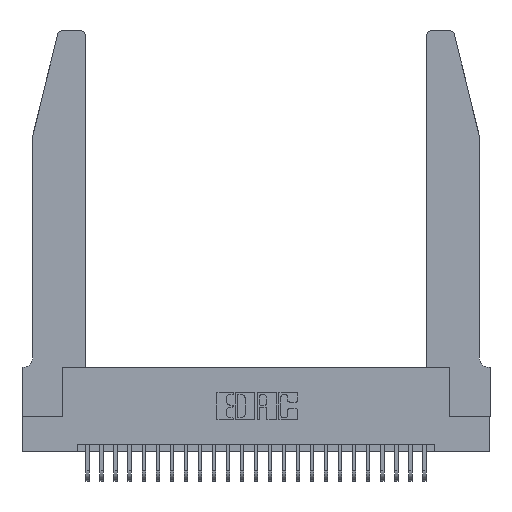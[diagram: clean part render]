
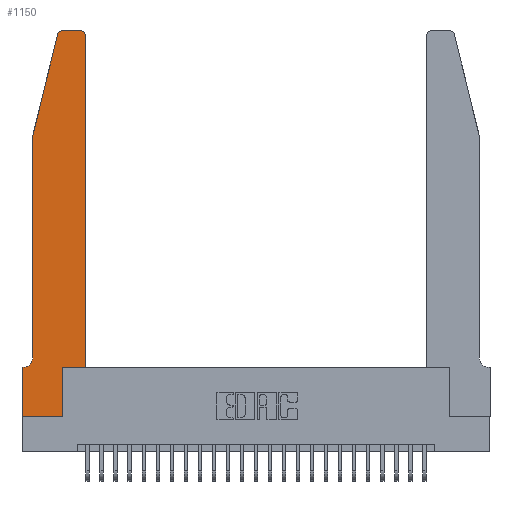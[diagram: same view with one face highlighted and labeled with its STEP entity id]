
A CAD part, top view. The second image highlights one B-rep face of the part: STEP entity #1150.
In plain terms, the highlighted planar face has unit normal (0, 0, 1).
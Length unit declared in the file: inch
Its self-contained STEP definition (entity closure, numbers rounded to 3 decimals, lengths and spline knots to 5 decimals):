
#134 = CARTESIAN_POINT ( 'NONE',  ( 0.2865, 0.35, 0.37 ) ) ;
#166 = ORIENTED_EDGE ( 'NONE', *, *, #511, .T. ) ;
#240 = CARTESIAN_POINT ( 'NONE',  ( 0.4205, 2.72, 0.37 ) ) ;
#432 = DIRECTION ( 'NONE',  ( 0., 0., 1. ) ) ;
#511 = EDGE_CURVE ( 'NONE', #27506, #2428, #8709, .T. ) ;
#896 = CARTESIAN_POINT ( 'NONE',  ( 0., 0., 0.37 ) ) ;
#1150 = ADVANCED_FACE ( 'NONE', ( #13424 ), #23059, .T. ) ;
#1518 = DIRECTION ( 'NONE',  ( 0., -1., 0. ) ) ;
#2144 = VERTEX_POINT ( 'NONE', #25174 ) ;
#2336 = VERTEX_POINT ( 'NONE', #21689 ) ;
#2428 = VERTEX_POINT ( 'NONE', #3837 ) ;
#2431 = CARTESIAN_POINT ( 'NONE',  ( 0., 0., 0.37 ) ) ;
#2516 = EDGE_CURVE ( 'NONE', #2428, #14756, #23964, .T. ) ;
#2703 = CARTESIAN_POINT ( 'NONE',  ( 0.2865, 0., 0.37 ) ) ;
#2908 = DIRECTION ( 'NONE',  ( 1., 0., 0. ) ) ;
#3651 = DIRECTION ( 'NONE',  ( -0.239, -0.971, 0. ) ) ;
#3837 = CARTESIAN_POINT ( 'NONE',  ( 0.4505, 0.35, 0.37 ) ) ;
#4097 = ORIENTED_EDGE ( 'NONE', *, *, #15264, .T. ) ;
#4547 = EDGE_CURVE ( 'NONE', #18676, #14718, #15716, .T. ) ;
#4570 = DIRECTION ( 'NONE',  ( 0., 1., 0. ) ) ;
#4845 = DIRECTION ( 'NONE',  ( 1., 0., 0. ) ) ;
#5157 = VERTEX_POINT ( 'NONE', #12170 ) ;
#5263 = DIRECTION ( 'NONE',  ( 1., 0., 0. ) ) ;
#5652 = DIRECTION ( 'NONE',  ( 1., 0., 0. ) ) ;
#6061 = LINE ( 'NONE', #9587, #26533 ) ;
#6070 = EDGE_CURVE ( 'NONE', #5157, #25349, #18004, .T. ) ;
#6197 = DIRECTION ( 'NONE',  ( 0., 0., 1. ) ) ;
#6421 = CARTESIAN_POINT ( 'NONE',  ( 0.4505, 0.35, 0.37 ) ) ;
#6541 = DIRECTION ( 'NONE',  ( 0., 1., 0. ) ) ;
#7028 = VECTOR ( 'NONE', #23090, 39.37008 ) ;
#7085 = ORIENTED_EDGE ( 'NONE', *, *, #6070, .T. ) ;
#7271 = VECTOR ( 'NONE', #4570, 39.37008 ) ;
#7482 = CARTESIAN_POINT ( 'NONE',  ( 0.2605, 2.75, 0.37 ) ) ;
#7517 = ORIENTED_EDGE ( 'NONE', *, *, #16308, .T. ) ;
#8447 = DIRECTION ( 'NONE',  ( 0., 0., -1. ) ) ;
#8467 = CARTESIAN_POINT ( 'NONE',  ( 0.4505, 0.35, 0.37 ) ) ;
#8530 = ORIENTED_EDGE ( 'NONE', *, *, #8780, .T. ) ;
#8709 = LINE ( 'NONE', #8467, #7028 ) ;
#8780 = EDGE_CURVE ( 'NONE', #25349, #9175, #27471, .T. ) ;
#9132 = ORIENTED_EDGE ( 'NONE', *, *, #11676, .T. ) ;
#9175 = VERTEX_POINT ( 'NONE', #12513 ) ;
#9546 = CARTESIAN_POINT ( 'NONE',  ( 0.284, 2.72, 0.37 ) ) ;
#9587 = CARTESIAN_POINT ( 'NONE',  ( 0.0755, 0.35, 0.37 ) ) ;
#9988 = EDGE_CURVE ( 'NONE', #22321, #27506, #17110, .T. ) ;
#10015 = CARTESIAN_POINT ( 'NONE',  ( 0., 0.35, 0.37 ) ) ;
#10237 = EDGE_CURVE ( 'NONE', #14718, #22321, #18480, .T. ) ;
#10330 = VECTOR ( 'NONE', #3651, 39.37008 ) ;
#10379 = CARTESIAN_POINT ( 'NONE',  ( 0.284, 2.75, 0.37 ) ) ;
#10900 = VECTOR ( 'NONE', #25086, 39.37008 ) ;
#11504 = CIRCLE ( 'NONE', #23195, 0.07 ) ;
#11676 = EDGE_CURVE ( 'NONE', #25065, #18676, #6061, .T. ) ;
#12170 = CARTESIAN_POINT ( 'NONE',  ( 0.4205, 2.75, 0.37 ) ) ;
#12513 = CARTESIAN_POINT ( 'NONE',  ( 0.25487, 2.72718, 0.37 ) ) ;
#12679 = LINE ( 'NONE', #18781, #23957 ) ;
#12920 = ORIENTED_EDGE ( 'NONE', *, *, #24057, .T. ) ;
#13315 = CARTESIAN_POINT ( 'NONE',  ( 0.4505, 2.72, 0.37 ) ) ;
#13424 = FACE_OUTER_BOUND ( 'NONE', #15771, .T. ) ;
#13601 = DIRECTION ( 'NONE',  ( 0., -1., 0. ) ) ;
#14072 = CARTESIAN_POINT ( 'NONE',  ( 0.0055, 0.35, 0.37 ) ) ;
#14718 = VERTEX_POINT ( 'NONE', #2431 ) ;
#14720 = LINE ( 'NONE', #16680, #10330 ) ;
#14756 = VERTEX_POINT ( 'NONE', #13315 ) ;
#15185 = ORIENTED_EDGE ( 'NONE', *, *, #26620, .T. ) ;
#15196 = ORIENTED_EDGE ( 'NONE', *, *, #9988, .T. ) ;
#15264 = EDGE_CURVE ( 'NONE', #9175, #2336, #14720, .T. ) ;
#15716 = LINE ( 'NONE', #896, #21188 ) ;
#15749 = VECTOR ( 'NONE', #5652, 39.37008 ) ;
#15771 = EDGE_LOOP ( 'NONE', ( #7085, #8530, #4097, #12920, #15185, #9132, #24798, #25247, #15196, #166, #18913, #7517 ) ) ;
#16308 = EDGE_CURVE ( 'NONE', #14756, #5157, #22179, .T. ) ;
#16680 = CARTESIAN_POINT ( 'NONE',  ( 0.0755, 2., 0.37 ) ) ;
#17110 = LINE ( 'NONE', #23765, #27079 ) ;
#18004 = LINE ( 'NONE', #7482, #10900 ) ;
#18480 = LINE ( 'NONE', #27620, #15749 ) ;
#18676 = VERTEX_POINT ( 'NONE', #26363 ) ;
#18781 = CARTESIAN_POINT ( 'NONE',  ( 0.0755, 2., 0.37 ) ) ;
#18913 = ORIENTED_EDGE ( 'NONE', *, *, #2516, .T. ) ;
#20431 = AXIS2_PLACEMENT_3D ( 'NONE', #10015, #25268, #5263 ) ;
#21188 = VECTOR ( 'NONE', #13601, 39.37008 ) ;
#21689 = CARTESIAN_POINT ( 'NONE',  ( 0.0755, 2., 0.37 ) ) ;
#22179 = CIRCLE ( 'NONE', #23954, 0.03 ) ;
#22321 = VERTEX_POINT ( 'NONE', #2703 ) ;
#23059 = PLANE ( 'NONE',  #20431 ) ;
#23090 = DIRECTION ( 'NONE',  ( 1., 0., 0. ) ) ;
#23195 = AXIS2_PLACEMENT_3D ( 'NONE', #25885, #8447, #27927 ) ;
#23765 = CARTESIAN_POINT ( 'NONE',  ( 0.2865, 0.35, 0.37 ) ) ;
#23954 = AXIS2_PLACEMENT_3D ( 'NONE', #240, #432, #4845 ) ;
#23957 = VECTOR ( 'NONE', #1518, 39.37008 ) ;
#23964 = LINE ( 'NONE', #6421, #7271 ) ;
#24057 = EDGE_CURVE ( 'NONE', #2336, #2144, #12679, .T. ) ;
#24798 = ORIENTED_EDGE ( 'NONE', *, *, #4547, .T. ) ;
#25065 = VERTEX_POINT ( 'NONE', #14072 ) ;
#25086 = DIRECTION ( 'NONE',  ( -1., 0., 0. ) ) ;
#25174 = CARTESIAN_POINT ( 'NONE',  ( 0.0755, 0.42, 0.37 ) ) ;
#25247 = ORIENTED_EDGE ( 'NONE', *, *, #10237, .T. ) ;
#25268 = DIRECTION ( 'NONE',  ( 0., 0., 1. ) ) ;
#25349 = VERTEX_POINT ( 'NONE', #10379 ) ;
#25885 = CARTESIAN_POINT ( 'NONE',  ( 0.0055, 0.42, 0.37 ) ) ;
#26286 = AXIS2_PLACEMENT_3D ( 'NONE', #9546, #6197, #2908 ) ;
#26363 = CARTESIAN_POINT ( 'NONE',  ( 0., 0.35, 0.37 ) ) ;
#26533 = VECTOR ( 'NONE', #27042, 39.37008 ) ;
#26620 = EDGE_CURVE ( 'NONE', #2144, #25065, #11504, .T. ) ;
#27042 = DIRECTION ( 'NONE',  ( -1., 0., 0. ) ) ;
#27079 = VECTOR ( 'NONE', #6541, 39.37008 ) ;
#27471 = CIRCLE ( 'NONE', #26286, 0.03 ) ;
#27506 = VERTEX_POINT ( 'NONE', #134 ) ;
#27620 = CARTESIAN_POINT ( 'NONE',  ( 0., 0., 0.37 ) ) ;
#27927 = DIRECTION ( 'NONE',  ( -1., 0., 0. ) ) ;
